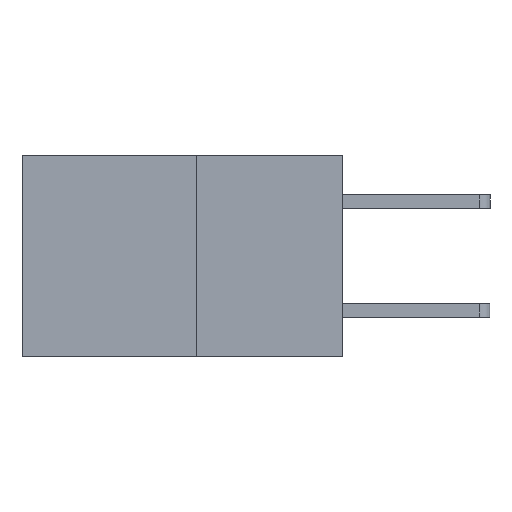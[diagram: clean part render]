
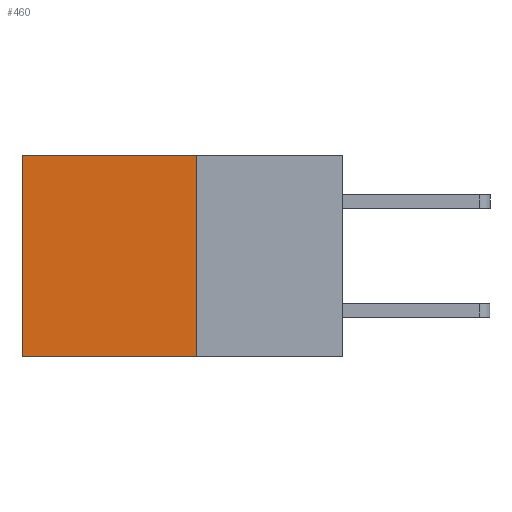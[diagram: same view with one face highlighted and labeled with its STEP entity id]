
A CAD part, left-side view. The second image highlights one B-rep face of the part: STEP entity #460.
In plain terms, the highlighted planar face has unit normal (-1, 0, 0).
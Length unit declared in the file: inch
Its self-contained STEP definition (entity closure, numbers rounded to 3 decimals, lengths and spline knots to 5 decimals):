
#19 = CARTESIAN_POINT ( 'NONE',  ( 0.277, 0.27, -0.37 ) ) ;
#97 = VECTOR ( 'NONE', #1024, 39.37008 ) ;
#460 = ADVANCED_FACE ( 'NONE', ( #6822 ), #7553, .F. ) ;
#514 = DIRECTION ( 'NONE',  ( 0., 1., 0. ) ) ;
#550 = CARTESIAN_POINT ( 'NONE',  ( 0.277, 0.27, -0.37 ) ) ;
#1024 = DIRECTION ( 'NONE',  ( 0., 1., 0. ) ) ;
#1028 = LINE ( 'NONE', #19, #5959 ) ;
#1485 = DIRECTION ( 'NONE',  ( 0., 0., -1. ) ) ;
#1812 = VECTOR ( 'NONE', #514, 39.37008 ) ;
#1941 = CARTESIAN_POINT ( 'NONE',  ( 0.277, 0.27, 0. ) ) ;
#2069 = EDGE_CURVE ( 'NONE', #6794, #5302, #6755, .T. ) ;
#2187 = LINE ( 'NONE', #550, #97 ) ;
#2770 = DIRECTION ( 'NONE',  ( 0., 0., -1. ) ) ;
#2810 = EDGE_CURVE ( 'NONE', #5302, #4419, #5484, .T. ) ;
#3132 = ORIENTED_EDGE ( 'NONE', *, *, #2810, .T. ) ;
#3774 = VECTOR ( 'NONE', #2770, 39.37008 ) ;
#4419 = VERTEX_POINT ( 'NONE', #5194 ) ;
#4842 = ORIENTED_EDGE ( 'NONE', *, *, #7171, .F. ) ;
#4884 = VERTEX_POINT ( 'NONE', #7247 ) ;
#5084 = CARTESIAN_POINT ( 'NONE',  ( 0.277, 0.59, -0.37 ) ) ;
#5094 = AXIS2_PLACEMENT_3D ( 'NONE', #7584, #7578, #7567 ) ;
#5194 = CARTESIAN_POINT ( 'NONE',  ( 0.277, 0.59, -0.37 ) ) ;
#5302 = VERTEX_POINT ( 'NONE', #5541 ) ;
#5484 = LINE ( 'NONE', #5084, #3774 ) ;
#5541 = CARTESIAN_POINT ( 'NONE',  ( 0.277, 0.59, 0. ) ) ;
#5959 = VECTOR ( 'NONE', #1485, 39.37008 ) ;
#6189 = EDGE_CURVE ( 'NONE', #6794, #4884, #1028, .T. ) ;
#6381 = ORIENTED_EDGE ( 'NONE', *, *, #6189, .F. ) ;
#6755 = LINE ( 'NONE', #1941, #1812 ) ;
#6794 = VERTEX_POINT ( 'NONE', #7223 ) ;
#6822 = FACE_OUTER_BOUND ( 'NONE', #7878, .T. ) ;
#7171 = EDGE_CURVE ( 'NONE', #4884, #4419, #2187, .T. ) ;
#7223 = CARTESIAN_POINT ( 'NONE',  ( 0.277, 0.27, 0. ) ) ;
#7247 = CARTESIAN_POINT ( 'NONE',  ( 0.277, 0.27, -0.37 ) ) ;
#7553 = PLANE ( 'NONE',  #5094 ) ;
#7567 = DIRECTION ( 'NONE',  ( 0., 0., -1. ) ) ;
#7578 = DIRECTION ( 'NONE',  ( 1., 0., 0. ) ) ;
#7584 = CARTESIAN_POINT ( 'NONE',  ( 0.277, 0.27, -0.37 ) ) ;
#7878 = EDGE_LOOP ( 'NONE', ( #3132, #4842, #6381, #7977 ) ) ;
#7977 = ORIENTED_EDGE ( 'NONE', *, *, #2069, .T. ) ;
